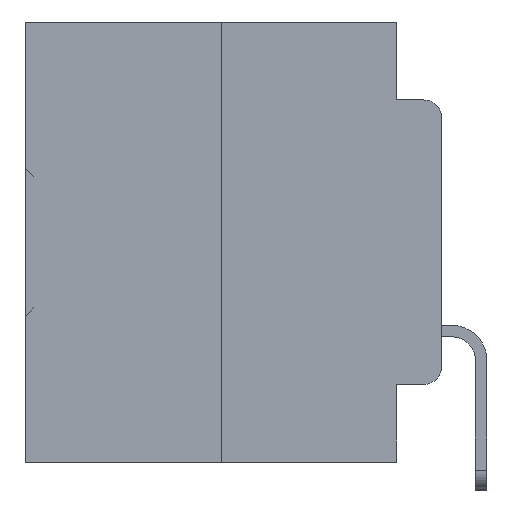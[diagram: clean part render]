
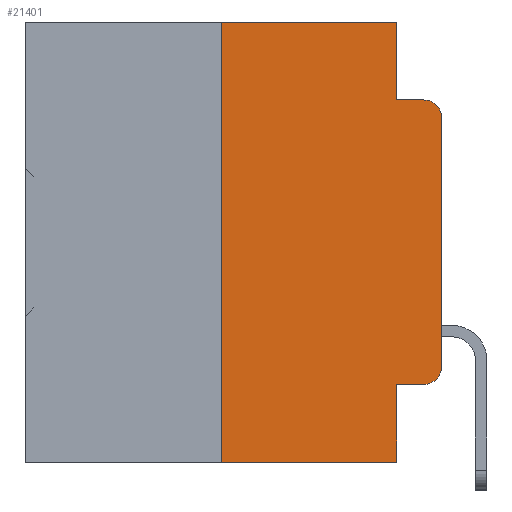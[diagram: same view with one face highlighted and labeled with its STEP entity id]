
A CAD part, left-side view. The second image highlights one B-rep face of the part: STEP entity #21401.
In plain terms, the highlighted planar face has unit normal (-1, 0, 0).
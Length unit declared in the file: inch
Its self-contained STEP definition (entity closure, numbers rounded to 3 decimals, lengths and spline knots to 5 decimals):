
#118 = LINE ( 'NONE', #19612, #35676 ) ;
#1604 = EDGE_LOOP ( 'NONE', ( #25479, #17747, #4328, #17435, #3985, #12010, #16542, #18471, #34013, #33020 ) ) ;
#2530 = CARTESIAN_POINT ( 'NONE',  ( 0., 0.051, -0.0885 ) ) ;
#2559 = FACE_OUTER_BOUND ( 'NONE', #1604, .T. ) ;
#2661 = DIRECTION ( 'NONE',  ( 0., -1., 0. ) ) ;
#3056 = EDGE_CURVE ( 'NONE', #9428, #3691, #32017, .T. ) ;
#3416 = CARTESIAN_POINT ( 'NONE',  ( 0., 0., -0.3915 ) ) ;
#3691 = VERTEX_POINT ( 'NONE', #30093 ) ;
#3985 = ORIENTED_EDGE ( 'NONE', *, *, #22744, .F. ) ;
#4201 = CARTESIAN_POINT ( 'NONE',  ( 0., 0.473, -0.5 ) ) ;
#4328 = ORIENTED_EDGE ( 'NONE', *, *, #30783, .F. ) ;
#4568 = CARTESIAN_POINT ( 'NONE',  ( 0., 0.051, -0.4115 ) ) ;
#4633 = VECTOR ( 'NONE', #16749, 39.37008 ) ;
#5561 = LINE ( 'NONE', #19670, #4633 ) ;
#8146 = DIRECTION ( 'NONE',  ( 0., 0., -1. ) ) ;
#8841 = VERTEX_POINT ( 'NONE', #37274 ) ;
#9428 = VERTEX_POINT ( 'NONE', #3416 ) ;
#9479 = VECTOR ( 'NONE', #2661, 39.37008 ) ;
#10915 = DIRECTION ( 'NONE',  ( 0., 0., -1. ) ) ;
#11146 = DIRECTION ( 'NONE',  ( -1., 0., 0. ) ) ;
#11361 = EDGE_CURVE ( 'NONE', #8841, #21696, #14069, .T. ) ;
#11548 = CARTESIAN_POINT ( 'NONE',  ( 0., 0.473, 0. ) ) ;
#11591 = EDGE_CURVE ( 'NONE', #18401, #9428, #21308, .T. ) ;
#11729 = CIRCLE ( 'NONE', #31803, 0.02 ) ;
#12010 = ORIENTED_EDGE ( 'NONE', *, *, #23182, .F. ) ;
#12277 = CARTESIAN_POINT ( 'NONE',  ( 0., 0.02, -0.4115 ) ) ;
#12400 = VERTEX_POINT ( 'NONE', #20861 ) ;
#13173 = VECTOR ( 'NONE', #18634, 39.37008 ) ;
#13200 = CARTESIAN_POINT ( 'NONE',  ( 0., 0.473, 0. ) ) ;
#13486 = EDGE_CURVE ( 'NONE', #27680, #18401, #17125, .T. ) ;
#13509 = AXIS2_PLACEMENT_3D ( 'NONE', #28328, #11146, #31194 ) ;
#13643 = CARTESIAN_POINT ( 'NONE',  ( 0., 0.02, -0.0885 ) ) ;
#14069 = LINE ( 'NONE', #4201, #13173 ) ;
#14414 = DIRECTION ( 'NONE',  ( 0., 0., -1. ) ) ;
#15463 = DIRECTION ( 'NONE',  ( -1., 0., 0. ) ) ;
#16542 = ORIENTED_EDGE ( 'NONE', *, *, #11361, .T. ) ;
#16749 = DIRECTION ( 'NONE',  ( 0., 0., 1. ) ) ;
#17125 = LINE ( 'NONE', #25638, #9479 ) ;
#17182 = CARTESIAN_POINT ( 'NONE',  ( 0., 0.051, -0.5 ) ) ;
#17435 = ORIENTED_EDGE ( 'NONE', *, *, #25076, .F. ) ;
#17747 = ORIENTED_EDGE ( 'NONE', *, *, #32672, .T. ) ;
#18401 = VERTEX_POINT ( 'NONE', #12277 ) ;
#18471 = ORIENTED_EDGE ( 'NONE', *, *, #21262, .F. ) ;
#18634 = DIRECTION ( 'NONE',  ( 0., -1., 0. ) ) ;
#18876 = CARTESIAN_POINT ( 'NONE',  ( 0., 0.051, -0.0885 ) ) ;
#19022 = DIRECTION ( 'NONE',  ( 0., -1., 0. ) ) ;
#19612 = CARTESIAN_POINT ( 'NONE',  ( 0., 0.051, 0. ) ) ;
#19670 = CARTESIAN_POINT ( 'NONE',  ( 0., 0.25, 0. ) ) ;
#20115 = VERTEX_POINT ( 'NONE', #31690 ) ;
#20861 = CARTESIAN_POINT ( 'NONE',  ( 0., 0.25, 0. ) ) ;
#21262 = EDGE_CURVE ( 'NONE', #27680, #21696, #22496, .T. ) ;
#21308 = CIRCLE ( 'NONE', #13509, 0.02 ) ;
#21401 = ADVANCED_FACE ( 'NONE', ( #2559 ), #25875, .F. ) ;
#21696 = VERTEX_POINT ( 'NONE', #17182 ) ;
#22496 = LINE ( 'NONE', #36622, #29168 ) ;
#22744 = EDGE_CURVE ( 'NONE', #12400, #20115, #28536, .T. ) ;
#23182 = EDGE_CURVE ( 'NONE', #8841, #12400, #5561, .T. ) ;
#24507 = VECTOR ( 'NONE', #27187, 39.37008 ) ;
#24944 = VECTOR ( 'NONE', #28504, 39.37008 ) ;
#25076 = EDGE_CURVE ( 'NONE', #20115, #35569, #118, .T. ) ;
#25479 = ORIENTED_EDGE ( 'NONE', *, *, #3056, .T. ) ;
#25638 = CARTESIAN_POINT ( 'NONE',  ( 0., 0.051, -0.4115 ) ) ;
#25875 = PLANE ( 'NONE',  #35313 ) ;
#27187 = DIRECTION ( 'NONE',  ( 0., 0., 1. ) ) ;
#27680 = VERTEX_POINT ( 'NONE', #4568 ) ;
#28328 = CARTESIAN_POINT ( 'NONE',  ( 0., 0.02, -0.3915 ) ) ;
#28504 = DIRECTION ( 'NONE',  ( 0., -1., 0. ) ) ;
#28536 = LINE ( 'NONE', #13200, #35162 ) ;
#29168 = VECTOR ( 'NONE', #10915, 39.37008 ) ;
#30093 = CARTESIAN_POINT ( 'NONE',  ( 0., 0., -0.1085 ) ) ;
#30116 = VERTEX_POINT ( 'NONE', #13643 ) ;
#30783 = EDGE_CURVE ( 'NONE', #35569, #30116, #33353, .T. ) ;
#31194 = DIRECTION ( 'NONE',  ( 0., 0., -1. ) ) ;
#31573 = DIRECTION ( 'NONE',  ( 1., 0., 0. ) ) ;
#31690 = CARTESIAN_POINT ( 'NONE',  ( 0., 0.051, 0. ) ) ;
#31803 = AXIS2_PLACEMENT_3D ( 'NONE', #32572, #15463, #35406 ) ;
#32017 = LINE ( 'NONE', #35586, #24507 ) ;
#32572 = CARTESIAN_POINT ( 'NONE',  ( 0., 0.02, -0.1085 ) ) ;
#32672 = EDGE_CURVE ( 'NONE', #3691, #30116, #11729, .T. ) ;
#33020 = ORIENTED_EDGE ( 'NONE', *, *, #11591, .T. ) ;
#33353 = LINE ( 'NONE', #2530, #24944 ) ;
#34013 = ORIENTED_EDGE ( 'NONE', *, *, #13486, .T. ) ;
#35162 = VECTOR ( 'NONE', #19022, 39.37008 ) ;
#35313 = AXIS2_PLACEMENT_3D ( 'NONE', #11548, #31573, #14414 ) ;
#35406 = DIRECTION ( 'NONE',  ( 0., 0., -1. ) ) ;
#35569 = VERTEX_POINT ( 'NONE', #18876 ) ;
#35586 = CARTESIAN_POINT ( 'NONE',  ( 0., 0., 0. ) ) ;
#35676 = VECTOR ( 'NONE', #8146, 39.37008 ) ;
#36622 = CARTESIAN_POINT ( 'NONE',  ( 0., 0.051, 0. ) ) ;
#37274 = CARTESIAN_POINT ( 'NONE',  ( 0., 0.25, -0.5 ) ) ;
